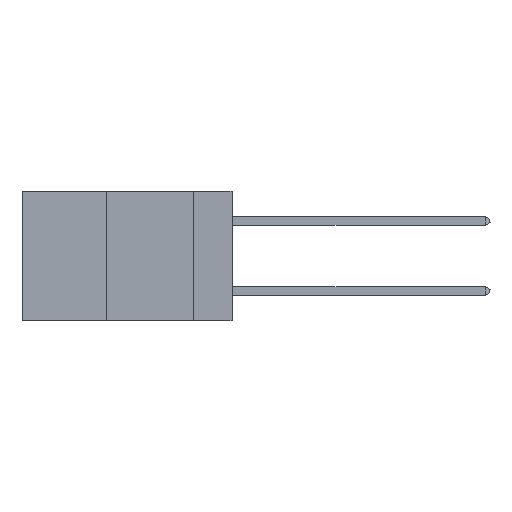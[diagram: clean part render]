
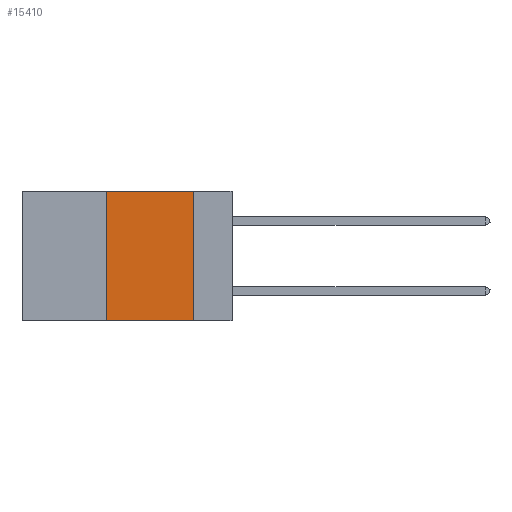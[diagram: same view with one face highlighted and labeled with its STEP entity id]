
A CAD part, left-side view. The second image highlights one B-rep face of the part: STEP entity #15410.
In plain terms, the highlighted planar face has unit normal (-1, 0, 0).
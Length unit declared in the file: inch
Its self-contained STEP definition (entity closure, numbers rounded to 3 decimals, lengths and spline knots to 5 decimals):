
#23 = EDGE_CURVE ( 'NONE', #21925, #659, #20847, .T. ) ;
#57 = CARTESIAN_POINT ( 'NONE',  ( 0., 0.36, -0.37 ) ) ;
#659 = VERTEX_POINT ( 'NONE', #12570 ) ;
#978 = VERTEX_POINT ( 'NONE', #57 ) ;
#1911 = VECTOR ( 'NONE', #12539, 39.37008 ) ;
#2050 = LINE ( 'NONE', #2087, #6717 ) ;
#2087 = CARTESIAN_POINT ( 'NONE',  ( 0., 0.6, -0.37 ) ) ;
#2772 = ORIENTED_EDGE ( 'NONE', *, *, #23, .F. ) ;
#2978 = PLANE ( 'NONE',  #17110 ) ;
#3697 = FACE_OUTER_BOUND ( 'NONE', #10207, .T. ) ;
#4991 = ORIENTED_EDGE ( 'NONE', *, *, #20116, .F. ) ;
#5385 = DIRECTION ( 'NONE',  ( 0., -1., 0. ) ) ;
#6717 = VECTOR ( 'NONE', #13117, 39.37008 ) ;
#6991 = DIRECTION ( 'NONE',  ( 1., 0., 0. ) ) ;
#8323 = CARTESIAN_POINT ( 'NONE',  ( 0., 0.36, 0. ) ) ;
#9470 = CARTESIAN_POINT ( 'NONE',  ( 0., 0.11, -0.37 ) ) ;
#9796 = CARTESIAN_POINT ( 'NONE',  ( 0., 0.6, 0. ) ) ;
#10207 = EDGE_LOOP ( 'NONE', ( #4991, #2772, #10765, #18266 ) ) ;
#10465 = CARTESIAN_POINT ( 'NONE',  ( 0., 0.6, 0. ) ) ;
#10765 = ORIENTED_EDGE ( 'NONE', *, *, #14166, .F. ) ;
#11047 = DIRECTION ( 'NONE',  ( 0., 0., -1. ) ) ;
#12539 = DIRECTION ( 'NONE',  ( 0., 0., 1. ) ) ;
#12570 = CARTESIAN_POINT ( 'NONE',  ( 0., 0.11, 0. ) ) ;
#13117 = DIRECTION ( 'NONE',  ( 0., -1., 0. ) ) ;
#14166 = EDGE_CURVE ( 'NONE', #978, #21925, #22492, .T. ) ;
#15410 = ADVANCED_FACE ( 'NONE', ( #3697 ), #2978, .F. ) ;
#15736 = LINE ( 'NONE', #20600, #20835 ) ;
#17019 = VERTEX_POINT ( 'NONE', #9470 ) ;
#17110 = AXIS2_PLACEMENT_3D ( 'NONE', #10465, #6991, #20435 ) ;
#18266 = ORIENTED_EDGE ( 'NONE', *, *, #23752, .T. ) ;
#20116 = EDGE_CURVE ( 'NONE', #659, #17019, #15736, .T. ) ;
#20225 = VECTOR ( 'NONE', #5385, 39.37008 ) ;
#20435 = DIRECTION ( 'NONE',  ( 0., 0., -1. ) ) ;
#20600 = CARTESIAN_POINT ( 'NONE',  ( 0., 0.11, 0. ) ) ;
#20835 = VECTOR ( 'NONE', #11047, 39.37008 ) ;
#20847 = LINE ( 'NONE', #9796, #20225 ) ;
#21925 = VERTEX_POINT ( 'NONE', #8323 ) ;
#22089 = CARTESIAN_POINT ( 'NONE',  ( 0., 0.36, 0. ) ) ;
#22492 = LINE ( 'NONE', #22089, #1911 ) ;
#23752 = EDGE_CURVE ( 'NONE', #978, #17019, #2050, .T. ) ;
